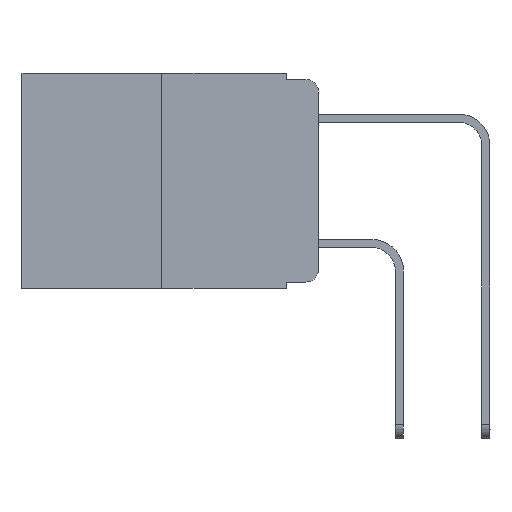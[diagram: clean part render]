
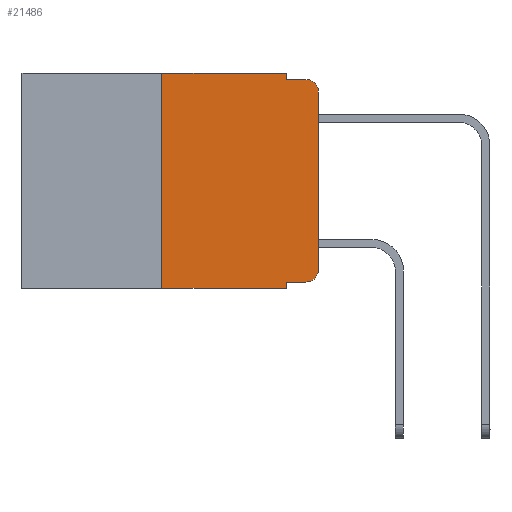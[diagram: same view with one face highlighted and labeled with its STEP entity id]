
A CAD part, left-side view. The second image highlights one B-rep face of the part: STEP entity #21486.
In plain terms, the highlighted planar face has unit normal (-1, 0, 0).
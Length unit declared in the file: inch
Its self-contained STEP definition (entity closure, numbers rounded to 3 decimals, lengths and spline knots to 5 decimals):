
#537 = ORIENTED_EDGE ( 'NONE', *, *, #16368, .T. ) ;
#907 = CARTESIAN_POINT ( 'NONE',  ( 0., 0.051, 0. ) ) ;
#1101 = CARTESIAN_POINT ( 'NONE',  ( 0., 0.02, -0.313 ) ) ;
#1244 = AXIS2_PLACEMENT_3D ( 'NONE', #8847, #7096, #1319 ) ;
#1261 = VERTEX_POINT ( 'NONE', #1846 ) ;
#1319 = DIRECTION ( 'NONE',  ( 0., 0., -1. ) ) ;
#1441 = CARTESIAN_POINT ( 'NONE',  ( 0., 0.051, 0. ) ) ;
#1846 = CARTESIAN_POINT ( 'NONE',  ( 0., 0.051, -0.01 ) ) ;
#1898 = VECTOR ( 'NONE', #24504, 39.37008 ) ;
#2014 = FACE_OUTER_BOUND ( 'NONE', #7314, .T. ) ;
#2288 = ORIENTED_EDGE ( 'NONE', *, *, #12827, .T. ) ;
#2826 = CARTESIAN_POINT ( 'NONE',  ( 0., 0.473, 0. ) ) ;
#2895 = ORIENTED_EDGE ( 'NONE', *, *, #15167, .F. ) ;
#3371 = DIRECTION ( 'NONE',  ( 0., -1., 0. ) ) ;
#3703 = AXIS2_PLACEMENT_3D ( 'NONE', #2826, #22073, #9000 ) ;
#3759 = LINE ( 'NONE', #20259, #22840 ) ;
#4798 = EDGE_CURVE ( 'NONE', #18441, #14165, #11830, .T. ) ;
#4864 = DIRECTION ( 'NONE',  ( 0., 0., 1. ) ) ;
#4938 = DIRECTION ( 'NONE',  ( 0., 0., -1. ) ) ;
#5615 = ORIENTED_EDGE ( 'NONE', *, *, #4798, .T. ) ;
#6180 = ORIENTED_EDGE ( 'NONE', *, *, #12834, .T. ) ;
#6341 = EDGE_CURVE ( 'NONE', #8257, #1261, #9077, .T. ) ;
#7096 = DIRECTION ( 'NONE',  ( -1., 0., 0. ) ) ;
#7314 = EDGE_LOOP ( 'NONE', ( #6180, #537, #15030, #21591, #12795, #18600, #5615, #2895, #19560, #2288 ) ) ;
#8257 = VERTEX_POINT ( 'NONE', #11728 ) ;
#8476 = CARTESIAN_POINT ( 'NONE',  ( 0., 0.02, -0.01 ) ) ;
#8754 = PLANE ( 'NONE',  #3703 ) ;
#8847 = CARTESIAN_POINT ( 'NONE',  ( 0., 0.02, -0.03 ) ) ;
#8969 = CARTESIAN_POINT ( 'NONE',  ( 0., 0., -0.313 ) ) ;
#9000 = DIRECTION ( 'NONE',  ( 0., 0., -1. ) ) ;
#9028 = LINE ( 'NONE', #23490, #14930 ) ;
#9077 = LINE ( 'NONE', #907, #18857 ) ;
#9360 = EDGE_CURVE ( 'NONE', #16474, #18644, #9028, .T. ) ;
#9409 = LINE ( 'NONE', #15018, #18019 ) ;
#10642 = VECTOR ( 'NONE', #19026, 39.37008 ) ;
#11106 = CARTESIAN_POINT ( 'NONE',  ( 0., 0.473, -0.343 ) ) ;
#11220 = CIRCLE ( 'NONE', #18733, 0.02 ) ;
#11361 = DIRECTION ( 'NONE',  ( 0., -1., 0. ) ) ;
#11728 = CARTESIAN_POINT ( 'NONE',  ( 0., 0.051, 0. ) ) ;
#11830 = LINE ( 'NONE', #11106, #21388 ) ;
#12050 = LINE ( 'NONE', #1441, #17700 ) ;
#12795 = ORIENTED_EDGE ( 'NONE', *, *, #24016, .F. ) ;
#12827 = EDGE_CURVE ( 'NONE', #18644, #22680, #11220, .T. ) ;
#12834 = EDGE_CURVE ( 'NONE', #22680, #14486, #3759, .T. ) ;
#12902 = EDGE_CURVE ( 'NONE', #18441, #20908, #21660, .T. ) ;
#14165 = VERTEX_POINT ( 'NONE', #17693 ) ;
#14486 = VERTEX_POINT ( 'NONE', #16974 ) ;
#14930 = VECTOR ( 'NONE', #19978, 39.37008 ) ;
#15018 = CARTESIAN_POINT ( 'NONE',  ( 0., 0.473, 0. ) ) ;
#15030 = ORIENTED_EDGE ( 'NONE', *, *, #15216, .F. ) ;
#15167 = EDGE_CURVE ( 'NONE', #16474, #14165, #12050, .T. ) ;
#15216 = EDGE_CURVE ( 'NONE', #1261, #24379, #15316, .T. ) ;
#15316 = LINE ( 'NONE', #16620, #1898 ) ;
#16368 = EDGE_CURVE ( 'NONE', #14486, #24379, #20972, .T. ) ;
#16474 = VERTEX_POINT ( 'NONE', #19346 ) ;
#16620 = CARTESIAN_POINT ( 'NONE',  ( 0., 0.051, -0.01 ) ) ;
#16923 = DIRECTION ( 'NONE',  ( 0., 0., -1. ) ) ;
#16974 = CARTESIAN_POINT ( 'NONE',  ( 0., 0., -0.03 ) ) ;
#17693 = CARTESIAN_POINT ( 'NONE',  ( 0., 0.051, -0.343 ) ) ;
#17700 = VECTOR ( 'NONE', #16923, 39.37008 ) ;
#18019 = VECTOR ( 'NONE', #11361, 39.37008 ) ;
#18401 = CARTESIAN_POINT ( 'NONE',  ( 0., 0.25, 0. ) ) ;
#18441 = VERTEX_POINT ( 'NONE', #20110 ) ;
#18600 = ORIENTED_EDGE ( 'NONE', *, *, #12902, .F. ) ;
#18644 = VERTEX_POINT ( 'NONE', #21564 ) ;
#18733 = AXIS2_PLACEMENT_3D ( 'NONE', #1101, #20076, #4938 ) ;
#18857 = VECTOR ( 'NONE', #21903, 39.37008 ) ;
#19026 = DIRECTION ( 'NONE',  ( 0., 0., 1. ) ) ;
#19346 = CARTESIAN_POINT ( 'NONE',  ( 0., 0.051, -0.333 ) ) ;
#19560 = ORIENTED_EDGE ( 'NONE', *, *, #9360, .T. ) ;
#19978 = DIRECTION ( 'NONE',  ( 0., -1., 0. ) ) ;
#20076 = DIRECTION ( 'NONE',  ( -1., 0., 0. ) ) ;
#20110 = CARTESIAN_POINT ( 'NONE',  ( 0., 0.25, -0.343 ) ) ;
#20259 = CARTESIAN_POINT ( 'NONE',  ( 0., 0., 0. ) ) ;
#20811 = CARTESIAN_POINT ( 'NONE',  ( 0., 0.25, 0. ) ) ;
#20908 = VERTEX_POINT ( 'NONE', #18401 ) ;
#20972 = CIRCLE ( 'NONE', #1244, 0.02 ) ;
#21388 = VECTOR ( 'NONE', #3371, 39.37008 ) ;
#21486 = ADVANCED_FACE ( 'NONE', ( #2014 ), #8754, .F. ) ;
#21564 = CARTESIAN_POINT ( 'NONE',  ( 0., 0.02, -0.333 ) ) ;
#21591 = ORIENTED_EDGE ( 'NONE', *, *, #6341, .F. ) ;
#21660 = LINE ( 'NONE', #20811, #10642 ) ;
#21903 = DIRECTION ( 'NONE',  ( 0., 0., -1. ) ) ;
#22073 = DIRECTION ( 'NONE',  ( 1., 0., 0. ) ) ;
#22680 = VERTEX_POINT ( 'NONE', #8969 ) ;
#22840 = VECTOR ( 'NONE', #4864, 39.37008 ) ;
#23490 = CARTESIAN_POINT ( 'NONE',  ( 0., 0.051, -0.333 ) ) ;
#24016 = EDGE_CURVE ( 'NONE', #20908, #8257, #9409, .T. ) ;
#24379 = VERTEX_POINT ( 'NONE', #8476 ) ;
#24504 = DIRECTION ( 'NONE',  ( 0., -1., 0. ) ) ;
